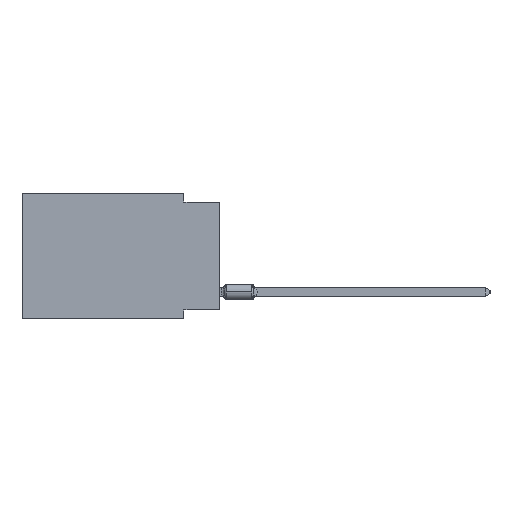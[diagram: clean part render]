
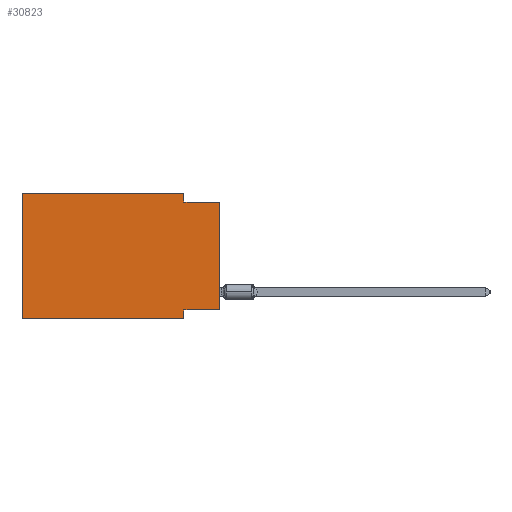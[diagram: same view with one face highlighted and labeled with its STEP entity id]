
A CAD part, left-side view. The second image highlights one B-rep face of the part: STEP entity #30823.
In plain terms, the highlighted planar face has unit normal (-1, 0, 0).
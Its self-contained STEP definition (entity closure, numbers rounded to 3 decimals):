
#112 = CARTESIAN_POINT ( 'NONE',  ( 0., 2.54, -8.89 ) ) ;
#298 = DIRECTION ( 'NONE',  ( 0., -1., 0. ) ) ;
#426 = EDGE_CURVE ( 'NONE', #39038, #8261, #17656, .T. ) ;
#1155 = VERTEX_POINT ( 'NONE', #23664 ) ;
#1715 = VERTEX_POINT ( 'NONE', #3648 ) ;
#1951 = CARTESIAN_POINT ( 'NONE',  ( 0., 0., -0.635 ) ) ;
#2354 = CARTESIAN_POINT ( 'NONE',  ( 0., 13.97, 0. ) ) ;
#3069 = DIRECTION ( 'NONE',  ( 0., -1., 0. ) ) ;
#3419 = CARTESIAN_POINT ( 'NONE',  ( 0., 2.54, 0. ) ) ;
#3648 = CARTESIAN_POINT ( 'NONE',  ( 0., 0., -8.255 ) ) ;
#4341 = VERTEX_POINT ( 'NONE', #1951 ) ;
#4402 = ORIENTED_EDGE ( 'NONE', *, *, #32534, .F. ) ;
#5507 = CARTESIAN_POINT ( 'NONE',  ( 0., 2.54, -0.635 ) ) ;
#6276 = VECTOR ( 'NONE', #23437, 1000. ) ;
#7606 = EDGE_CURVE ( 'NONE', #36139, #4341, #30755, .T. ) ;
#8261 = VERTEX_POINT ( 'NONE', #3419 ) ;
#9069 = FACE_OUTER_BOUND ( 'NONE', #30187, .T. ) ;
#9594 = CARTESIAN_POINT ( 'NONE',  ( 0., 2.54, 0. ) ) ;
#10241 = CARTESIAN_POINT ( 'NONE',  ( 0., 0., 0. ) ) ;
#10251 = LINE ( 'NONE', #14143, #18165 ) ;
#10408 = LINE ( 'NONE', #17674, #47436 ) ;
#10838 = CARTESIAN_POINT ( 'NONE',  ( 0., 2.54, -8.255 ) ) ;
#11111 = ORIENTED_EDGE ( 'NONE', *, *, #18283, .F. ) ;
#11450 = VERTEX_POINT ( 'NONE', #112 ) ;
#12191 = EDGE_CURVE ( 'NONE', #1155, #39038, #10408, .T. ) ;
#12767 = LINE ( 'NONE', #9594, #29974 ) ;
#12970 = PLANE ( 'NONE',  #34396 ) ;
#13053 = EDGE_CURVE ( 'NONE', #1155, #11450, #37285, .T. ) ;
#14143 = CARTESIAN_POINT ( 'NONE',  ( 0., 0., -8.255 ) ) ;
#16771 = VERTEX_POINT ( 'NONE', #10838 ) ;
#17251 = ORIENTED_EDGE ( 'NONE', *, *, #33109, .F. ) ;
#17656 = LINE ( 'NONE', #2354, #39047 ) ;
#17674 = CARTESIAN_POINT ( 'NONE',  ( 0., 13.97, 0. ) ) ;
#18165 = VECTOR ( 'NONE', #43110, 1000. ) ;
#18213 = CARTESIAN_POINT ( 'NONE',  ( 0., 13.97, 0. ) ) ;
#18283 = EDGE_CURVE ( 'NONE', #8261, #36139, #12767, .T. ) ;
#18789 = CARTESIAN_POINT ( 'NONE',  ( 0., 13.97, -8.89 ) ) ;
#20694 = DIRECTION ( 'NONE',  ( 0., 0., 1. ) ) ;
#21714 = VECTOR ( 'NONE', #29893, 1000. ) ;
#23345 = ORIENTED_EDGE ( 'NONE', *, *, #12191, .F. ) ;
#23437 = DIRECTION ( 'NONE',  ( 0., -1., 0. ) ) ;
#23664 = CARTESIAN_POINT ( 'NONE',  ( 0., 13.97, -8.89 ) ) ;
#25100 = VECTOR ( 'NONE', #20694, 1000. ) ;
#27376 = ORIENTED_EDGE ( 'NONE', *, *, #7606, .F. ) ;
#28140 = ORIENTED_EDGE ( 'NONE', *, *, #13053, .T. ) ;
#28316 = DIRECTION ( 'NONE',  ( 0., 0., -1. ) ) ;
#29893 = DIRECTION ( 'NONE',  ( 0., 0., -1. ) ) ;
#29974 = VECTOR ( 'NONE', #28316, 1000. ) ;
#30187 = EDGE_LOOP ( 'NONE', ( #32148, #27376, #11111, #34342, #23345, #28140, #17251, #4402 ) ) ;
#30755 = LINE ( 'NONE', #41483, #6276 ) ;
#30823 = ADVANCED_FACE ( 'NONE', ( #9069 ), #12970, .F. ) ;
#31328 = EDGE_CURVE ( 'NONE', #1715, #4341, #38001, .T. ) ;
#32148 = ORIENTED_EDGE ( 'NONE', *, *, #31328, .T. ) ;
#32534 = EDGE_CURVE ( 'NONE', #1715, #16771, #10251, .T. ) ;
#33062 = CARTESIAN_POINT ( 'NONE',  ( 0., 2.54, -8.89 ) ) ;
#33109 = EDGE_CURVE ( 'NONE', #16771, #11450, #40599, .T. ) ;
#34342 = ORIENTED_EDGE ( 'NONE', *, *, #426, .F. ) ;
#34396 = AXIS2_PLACEMENT_3D ( 'NONE', #34653, #42423, #46081 ) ;
#34653 = CARTESIAN_POINT ( 'NONE',  ( 0., 13.97, 0. ) ) ;
#36139 = VERTEX_POINT ( 'NONE', #5507 ) ;
#37285 = LINE ( 'NONE', #18789, #37403 ) ;
#37403 = VECTOR ( 'NONE', #298, 1000. ) ;
#38001 = LINE ( 'NONE', #10241, #25100 ) ;
#39038 = VERTEX_POINT ( 'NONE', #18213 ) ;
#39047 = VECTOR ( 'NONE', #3069, 1000. ) ;
#40599 = LINE ( 'NONE', #33062, #21714 ) ;
#41483 = CARTESIAN_POINT ( 'NONE',  ( 0., 0., -0.635 ) ) ;
#42423 = DIRECTION ( 'NONE',  ( 1., 0., 0. ) ) ;
#42781 = DIRECTION ( 'NONE',  ( 0., 0., 1. ) ) ;
#43110 = DIRECTION ( 'NONE',  ( 0., 1., 0. ) ) ;
#46081 = DIRECTION ( 'NONE',  ( 0., 0., -1. ) ) ;
#47436 = VECTOR ( 'NONE', #42781, 1000. ) ;
